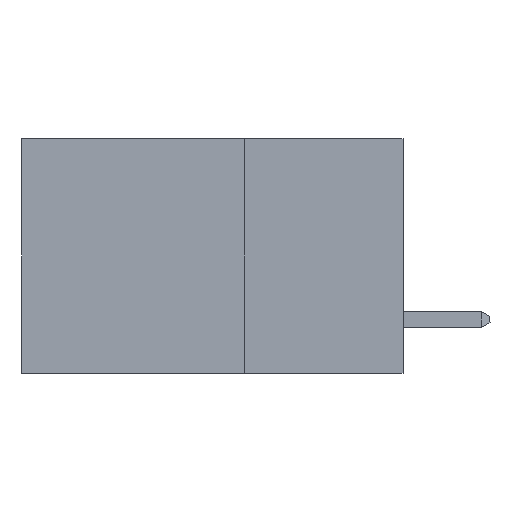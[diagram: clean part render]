
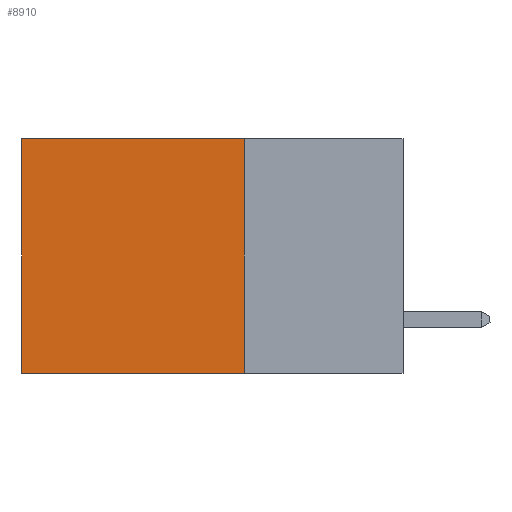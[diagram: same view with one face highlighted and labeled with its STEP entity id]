
A CAD part, left-side view. The second image highlights one B-rep face of the part: STEP entity #8910.
In plain terms, the highlighted planar face has unit normal (-1, 0, 0).
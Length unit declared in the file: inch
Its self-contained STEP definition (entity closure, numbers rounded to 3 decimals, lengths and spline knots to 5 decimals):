
#498 = ORIENTED_EDGE ( 'NONE', *, *, #10545, .F. ) ;
#1662 = VERTEX_POINT ( 'NONE', #6065 ) ;
#1801 = LINE ( 'NONE', #9162, #6372 ) ;
#2187 = CARTESIAN_POINT ( 'NONE',  ( 0.2875, 0.25, 0. ) ) ;
#2764 = LINE ( 'NONE', #16534, #12779 ) ;
#4116 = VECTOR ( 'NONE', #9310, 39.37008 ) ;
#4607 = VECTOR ( 'NONE', #20679, 39.37008 ) ;
#5062 = ORIENTED_EDGE ( 'NONE', *, *, #23508, .T. ) ;
#5190 = CARTESIAN_POINT ( 'NONE',  ( 0.2875, 0.6, 0. ) ) ;
#5229 = LINE ( 'NONE', #22489, #4607 ) ;
#5398 = EDGE_CURVE ( 'NONE', #12898, #1662, #2764, .T. ) ;
#5467 = DIRECTION ( 'NONE',  ( 0., 0., -1. ) ) ;
#6065 = CARTESIAN_POINT ( 'NONE',  ( 0.2875, 0.25, -0.37 ) ) ;
#6372 = VECTOR ( 'NONE', #12858, 39.37008 ) ;
#7440 = CARTESIAN_POINT ( 'NONE',  ( 0.2875, 0.25, -0.37 ) ) ;
#7989 = PLANE ( 'NONE',  #17604 ) ;
#8910 = ADVANCED_FACE ( 'NONE', ( #18072 ), #7989, .F. ) ;
#9162 = CARTESIAN_POINT ( 'NONE',  ( 0.2875, 0.25, 0. ) ) ;
#9310 = DIRECTION ( 'NONE',  ( 0., 1., 0. ) ) ;
#9860 = DIRECTION ( 'NONE',  ( 0., 0., -1. ) ) ;
#10545 = EDGE_CURVE ( 'NONE', #1662, #18387, #18901, .T. ) ;
#11509 = EDGE_LOOP ( 'NONE', ( #5062, #498, #20286, #20169 ) ) ;
#12301 = VERTEX_POINT ( 'NONE', #5190 ) ;
#12373 = CARTESIAN_POINT ( 'NONE',  ( 0.2875, 0.6, -0.37 ) ) ;
#12779 = VECTOR ( 'NONE', #5467, 39.37008 ) ;
#12858 = DIRECTION ( 'NONE',  ( 0., 1., 0. ) ) ;
#12898 = VERTEX_POINT ( 'NONE', #23448 ) ;
#12986 = EDGE_CURVE ( 'NONE', #12898, #12301, #1801, .T. ) ;
#16534 = CARTESIAN_POINT ( 'NONE',  ( 0.2875, 0.25, 0. ) ) ;
#17604 = AXIS2_PLACEMENT_3D ( 'NONE', #2187, #20822, #9860 ) ;
#18072 = FACE_OUTER_BOUND ( 'NONE', #11509, .T. ) ;
#18387 = VERTEX_POINT ( 'NONE', #12373 ) ;
#18901 = LINE ( 'NONE', #7440, #4116 ) ;
#20169 = ORIENTED_EDGE ( 'NONE', *, *, #12986, .T. ) ;
#20286 = ORIENTED_EDGE ( 'NONE', *, *, #5398, .F. ) ;
#20679 = DIRECTION ( 'NONE',  ( 0., 0., -1. ) ) ;
#20822 = DIRECTION ( 'NONE',  ( 1., 0., 0. ) ) ;
#22489 = CARTESIAN_POINT ( 'NONE',  ( 0.2875, 0.6, 0. ) ) ;
#23448 = CARTESIAN_POINT ( 'NONE',  ( 0.2875, 0.25, 0. ) ) ;
#23508 = EDGE_CURVE ( 'NONE', #12301, #18387, #5229, .T. ) ;
